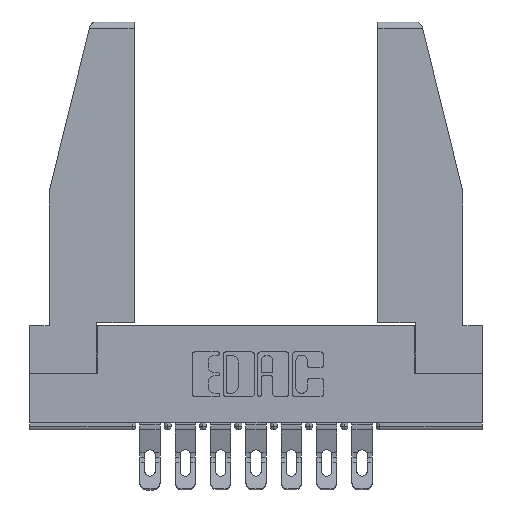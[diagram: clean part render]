
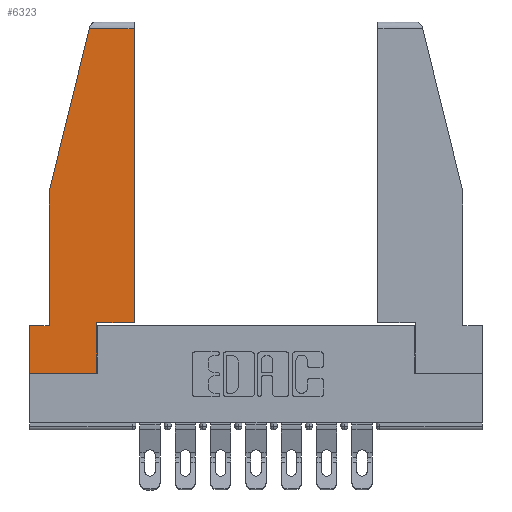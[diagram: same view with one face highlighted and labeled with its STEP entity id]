
A CAD part, top view. The second image highlights one B-rep face of the part: STEP entity #6323.
In plain terms, the highlighted planar face has unit normal (0, 0, 1).
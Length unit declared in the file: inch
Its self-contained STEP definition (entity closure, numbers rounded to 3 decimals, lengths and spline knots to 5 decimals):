
#262 = VECTOR ( 'NONE', #4108, 39.37008 ) ;
#529 = CARTESIAN_POINT ( 'NONE',  ( 0.461, 0.223, 0. ) ) ;
#534 = LINE ( 'NONE', #1788, #10574 ) ;
#705 = ORIENTED_EDGE ( 'NONE', *, *, #3161, .T. ) ;
#761 = PLANE ( 'NONE',  #12464 ) ;
#858 = CARTESIAN_POINT ( 'NONE',  ( 0., 0., 0. ) ) ;
#920 = CARTESIAN_POINT ( 'NONE',  ( 0.086, 0.21, 0. ) ) ;
#991 = LINE ( 'NONE', #3692, #7107 ) ;
#1075 = FACE_OUTER_BOUND ( 'NONE', #6993, .T. ) ;
#1788 = CARTESIAN_POINT ( 'NONE',  ( 0.297, 0.223, 0. ) ) ;
#1929 = CARTESIAN_POINT ( 'NONE',  ( 0., 0., 0. ) ) ;
#2302 = VECTOR ( 'NONE', #10628, 39.37008 ) ;
#2405 = CARTESIAN_POINT ( 'NONE',  ( 0.086, 0.8, 0. ) ) ;
#2925 = DIRECTION ( 'NONE',  ( 1., 0., 0. ) ) ;
#3136 = CARTESIAN_POINT ( 'NONE',  ( 0.297, 0., 0. ) ) ;
#3143 = VERTEX_POINT ( 'NONE', #2405 ) ;
#3161 = EDGE_CURVE ( 'NONE', #13838, #3143, #5635, .T. ) ;
#3328 = VERTEX_POINT ( 'NONE', #920 ) ;
#3335 = VERTEX_POINT ( 'NONE', #6727 ) ;
#3692 = CARTESIAN_POINT ( 'NONE',  ( 0.461, 0.223, 0. ) ) ;
#3756 = DIRECTION ( 'NONE',  ( 0., -1., 0. ) ) ;
#4000 = VECTOR ( 'NONE', #10772, 39.37008 ) ;
#4108 = DIRECTION ( 'NONE',  ( -1., 0., 0. ) ) ;
#4509 = EDGE_CURVE ( 'NONE', #10911, #10906, #10436, .T. ) ;
#4690 = VECTOR ( 'NONE', #9935, 39.37008 ) ;
#4835 = VERTEX_POINT ( 'NONE', #7765 ) ;
#5081 = EDGE_CURVE ( 'NONE', #3143, #3328, #11333, .T. ) ;
#5353 = LINE ( 'NONE', #9472, #2302 ) ;
#5625 = ORIENTED_EDGE ( 'NONE', *, *, #5081, .T. ) ;
#5635 = LINE ( 'NONE', #8165, #9217 ) ;
#5896 = ORIENTED_EDGE ( 'NONE', *, *, #7094, .T. ) ;
#6004 = DIRECTION ( 'NONE',  ( 0., 1., 0. ) ) ;
#6208 = VECTOR ( 'NONE', #6449, 39.37008 ) ;
#6323 = ADVANCED_FACE ( 'NONE', ( #1075 ), #761, .T. ) ;
#6449 = DIRECTION ( 'NONE',  ( 0., 1., 0. ) ) ;
#6519 = EDGE_CURVE ( 'NONE', #8761, #11620, #534, .T. ) ;
#6630 = CARTESIAN_POINT ( 'NONE',  ( 0., 0.21, 0. ) ) ;
#6727 = CARTESIAN_POINT ( 'NONE',  ( 0., 0.21, 0. ) ) ;
#6993 = EDGE_LOOP ( 'NONE', ( #12003, #5896, #705, #5625, #12573, #8052, #13917, #12988, #8484 ) ) ;
#7094 = EDGE_CURVE ( 'NONE', #4835, #13838, #5353, .T. ) ;
#7107 = VECTOR ( 'NONE', #6004, 39.37008 ) ;
#7717 = CARTESIAN_POINT ( 'NONE',  ( 0., 0., 0. ) ) ;
#7765 = CARTESIAN_POINT ( 'NONE',  ( 0.461, 1.52, 0. ) ) ;
#8052 = ORIENTED_EDGE ( 'NONE', *, *, #14162, .T. ) ;
#8136 = CARTESIAN_POINT ( 'NONE',  ( 0., 0.21, 0. ) ) ;
#8160 = LINE ( 'NONE', #3136, #6208 ) ;
#8165 = CARTESIAN_POINT ( 'NONE',  ( 0.271, 1.55, 0. ) ) ;
#8460 = EDGE_CURVE ( 'NONE', #11620, #4835, #991, .T. ) ;
#8484 = ORIENTED_EDGE ( 'NONE', *, *, #6519, .T. ) ;
#8761 = VERTEX_POINT ( 'NONE', #10573 ) ;
#8908 = DIRECTION ( 'NONE',  ( 0., 0., 1. ) ) ;
#9217 = VECTOR ( 'NONE', #11580, 39.37008 ) ;
#9472 = CARTESIAN_POINT ( 'NONE',  ( 0., 1.52, 0. ) ) ;
#9935 = DIRECTION ( 'NONE',  ( 1., 0., 0. ) ) ;
#10436 = LINE ( 'NONE', #1929, #4690 ) ;
#10573 = CARTESIAN_POINT ( 'NONE',  ( 0.297, 0.223, 0. ) ) ;
#10574 = VECTOR ( 'NONE', #2925, 39.37008 ) ;
#10628 = DIRECTION ( 'NONE',  ( -1., 0., 0. ) ) ;
#10772 = DIRECTION ( 'NONE',  ( 0., -1., 0. ) ) ;
#10906 = VERTEX_POINT ( 'NONE', #14771 ) ;
#10911 = VERTEX_POINT ( 'NONE', #7717 ) ;
#11018 = DIRECTION ( 'NONE',  ( 1., 0., 0. ) ) ;
#11333 = LINE ( 'NONE', #12527, #14774 ) ;
#11580 = DIRECTION ( 'NONE',  ( -0.239, -0.971, 0. ) ) ;
#11620 = VERTEX_POINT ( 'NONE', #529 ) ;
#11961 = LINE ( 'NONE', #8136, #4000 ) ;
#12003 = ORIENTED_EDGE ( 'NONE', *, *, #8460, .T. ) ;
#12322 = EDGE_CURVE ( 'NONE', #10906, #8761, #8160, .T. ) ;
#12464 = AXIS2_PLACEMENT_3D ( 'NONE', #858, #8908, #11018 ) ;
#12514 = LINE ( 'NONE', #6630, #262 ) ;
#12527 = CARTESIAN_POINT ( 'NONE',  ( 0.086, 0.8, 0. ) ) ;
#12573 = ORIENTED_EDGE ( 'NONE', *, *, #13803, .T. ) ;
#12988 = ORIENTED_EDGE ( 'NONE', *, *, #12322, .T. ) ;
#13514 = CARTESIAN_POINT ( 'NONE',  ( 0.2636, 1.52, 0. ) ) ;
#13803 = EDGE_CURVE ( 'NONE', #3328, #3335, #12514, .T. ) ;
#13838 = VERTEX_POINT ( 'NONE', #13514 ) ;
#13917 = ORIENTED_EDGE ( 'NONE', *, *, #4509, .T. ) ;
#14162 = EDGE_CURVE ( 'NONE', #3335, #10911, #11961, .T. ) ;
#14771 = CARTESIAN_POINT ( 'NONE',  ( 0.297, 0., 0. ) ) ;
#14774 = VECTOR ( 'NONE', #3756, 39.37008 ) ;
